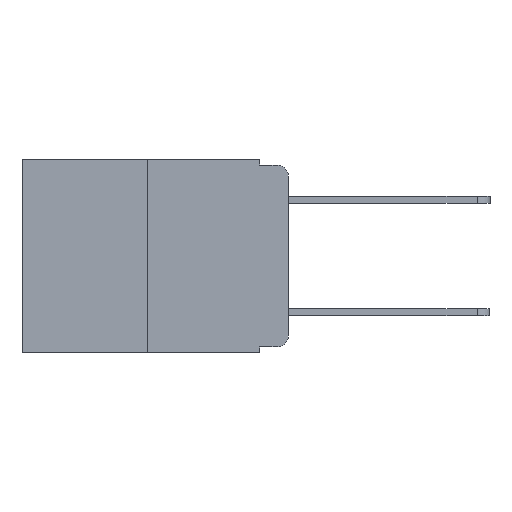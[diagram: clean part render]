
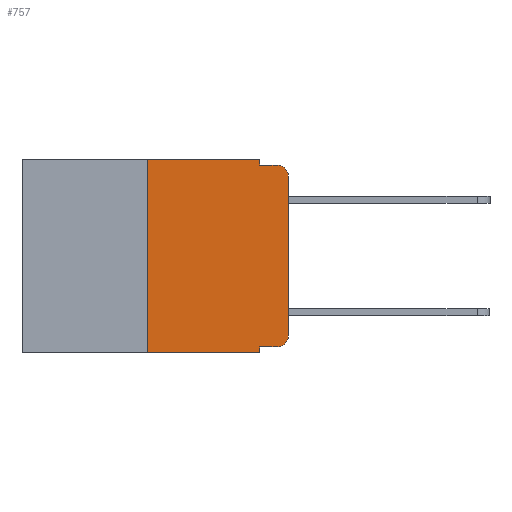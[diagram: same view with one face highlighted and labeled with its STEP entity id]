
A CAD part, left-side view. The second image highlights one B-rep face of the part: STEP entity #757.
In plain terms, the highlighted planar face has unit normal (-1, 0, 0).
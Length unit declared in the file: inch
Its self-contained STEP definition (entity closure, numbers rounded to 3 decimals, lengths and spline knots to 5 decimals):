
#207 = VERTEX_POINT ( 'NONE', #7604 ) ;
#757 = ADVANCED_FACE ( 'NONE', ( #16403 ), #2458, .F. ) ;
#1333 = CARTESIAN_POINT ( 'NONE',  ( 0., 0.02, -0.313 ) ) ;
#1592 = ORIENTED_EDGE ( 'NONE', *, *, #16100, .T. ) ;
#1748 = EDGE_CURVE ( 'NONE', #19135, #207, #5125, .T. ) ;
#2001 = VERTEX_POINT ( 'NONE', #13512 ) ;
#2207 = ORIENTED_EDGE ( 'NONE', *, *, #8407, .F. ) ;
#2458 = PLANE ( 'NONE',  #22875 ) ;
#2484 = AXIS2_PLACEMENT_3D ( 'NONE', #18502, #7836, #20227 ) ;
#2815 = CARTESIAN_POINT ( 'NONE',  ( 0., 0.051, -0.343 ) ) ;
#3214 = DIRECTION ( 'NONE',  ( 0., 0., -1. ) ) ;
#3325 = VECTOR ( 'NONE', #6376, 39.37008 ) ;
#3663 = EDGE_CURVE ( 'NONE', #4426, #10604, #8149, .T. ) ;
#3770 = ORIENTED_EDGE ( 'NONE', *, *, #12910, .T. ) ;
#4057 = LINE ( 'NONE', #16016, #12547 ) ;
#4163 = CIRCLE ( 'NONE', #2484, 0.02 ) ;
#4196 = CARTESIAN_POINT ( 'NONE',  ( 0., 0.25, -0.343 ) ) ;
#4425 = EDGE_CURVE ( 'NONE', #16785, #2001, #16792, .T. ) ;
#4426 = VERTEX_POINT ( 'NONE', #22706 ) ;
#4453 = CARTESIAN_POINT ( 'NONE',  ( 0., 0., -0.03 ) ) ;
#4500 = LINE ( 'NONE', #19977, #8775 ) ;
#4833 = VERTEX_POINT ( 'NONE', #6075 ) ;
#5109 = LINE ( 'NONE', #6701, #14104 ) ;
#5125 = LINE ( 'NONE', #15799, #9956 ) ;
#5719 = DIRECTION ( 'NONE',  ( 0., 0., -1. ) ) ;
#5805 = VECTOR ( 'NONE', #20766, 39.37008 ) ;
#6075 = CARTESIAN_POINT ( 'NONE',  ( 0., 0.02, -0.01 ) ) ;
#6245 = ORIENTED_EDGE ( 'NONE', *, *, #14078, .T. ) ;
#6376 = DIRECTION ( 'NONE',  ( 0., 0., -1. ) ) ;
#6575 = CARTESIAN_POINT ( 'NONE',  ( 0., 0., 0. ) ) ;
#6591 = EDGE_CURVE ( 'NONE', #14006, #4833, #12636, .T. ) ;
#6701 = CARTESIAN_POINT ( 'NONE',  ( 0., 0.473, -0.343 ) ) ;
#6834 = VERTEX_POINT ( 'NONE', #4453 ) ;
#7321 = CARTESIAN_POINT ( 'NONE',  ( 0., 0.051, -0.01 ) ) ;
#7604 = CARTESIAN_POINT ( 'NONE',  ( 0., 0.25, 0. ) ) ;
#7836 = DIRECTION ( 'NONE',  ( -1., 0., 0. ) ) ;
#8149 = LINE ( 'NONE', #17876, #3325 ) ;
#8407 = EDGE_CURVE ( 'NONE', #22431, #14006, #4057, .T. ) ;
#8775 = VECTOR ( 'NONE', #11318, 39.37008 ) ;
#9539 = ORIENTED_EDGE ( 'NONE', *, *, #22775, .F. ) ;
#9803 = CARTESIAN_POINT ( 'NONE',  ( 0., 0.473, 0. ) ) ;
#9956 = VECTOR ( 'NONE', #10819, 39.37008 ) ;
#10178 = EDGE_CURVE ( 'NONE', #19135, #10604, #5109, .T. ) ;
#10604 = VERTEX_POINT ( 'NONE', #2815 ) ;
#10627 = LINE ( 'NONE', #6575, #5805 ) ;
#10819 = DIRECTION ( 'NONE',  ( 0., 0., 1. ) ) ;
#11318 = DIRECTION ( 'NONE',  ( 0., -1., 0. ) ) ;
#11616 = DIRECTION ( 'NONE',  ( 0., -1., 0. ) ) ;
#12024 = ORIENTED_EDGE ( 'NONE', *, *, #3663, .F. ) ;
#12097 = VECTOR ( 'NONE', #12846, 39.37008 ) ;
#12169 = DIRECTION ( 'NONE',  ( 0., -1., 0. ) ) ;
#12547 = VECTOR ( 'NONE', #17937, 39.37008 ) ;
#12636 = LINE ( 'NONE', #7321, #12097 ) ;
#12750 = CARTESIAN_POINT ( 'NONE',  ( 0., 0.051, 0. ) ) ;
#12846 = DIRECTION ( 'NONE',  ( 0., -1., 0. ) ) ;
#12910 = EDGE_CURVE ( 'NONE', #4426, #16785, #4500, .T. ) ;
#12916 = ORIENTED_EDGE ( 'NONE', *, *, #1748, .F. ) ;
#13512 = CARTESIAN_POINT ( 'NONE',  ( 0., 0., -0.313 ) ) ;
#13540 = ORIENTED_EDGE ( 'NONE', *, *, #6591, .F. ) ;
#14005 = DIRECTION ( 'NONE',  ( -1., 0., 0. ) ) ;
#14006 = VERTEX_POINT ( 'NONE', #19926 ) ;
#14078 = EDGE_CURVE ( 'NONE', #6834, #4833, #4163, .T. ) ;
#14104 = VECTOR ( 'NONE', #12169, 39.37008 ) ;
#14227 = ORIENTED_EDGE ( 'NONE', *, *, #4425, .T. ) ;
#15799 = CARTESIAN_POINT ( 'NONE',  ( 0., 0.25, 0. ) ) ;
#16016 = CARTESIAN_POINT ( 'NONE',  ( 0., 0.051, 0. ) ) ;
#16100 = EDGE_CURVE ( 'NONE', #2001, #6834, #10627, .T. ) ;
#16403 = FACE_OUTER_BOUND ( 'NONE', #19066, .T. ) ;
#16785 = VERTEX_POINT ( 'NONE', #21453 ) ;
#16792 = CIRCLE ( 'NONE', #18140, 0.02 ) ;
#17295 = CARTESIAN_POINT ( 'NONE',  ( 0., 0.473, 0. ) ) ;
#17876 = CARTESIAN_POINT ( 'NONE',  ( 0., 0.051, 0. ) ) ;
#17937 = DIRECTION ( 'NONE',  ( 0., 0., -1. ) ) ;
#18140 = AXIS2_PLACEMENT_3D ( 'NONE', #1333, #14005, #3214 ) ;
#18502 = CARTESIAN_POINT ( 'NONE',  ( 0., 0.02, -0.03 ) ) ;
#19066 = EDGE_LOOP ( 'NONE', ( #1592, #6245, #13540, #2207, #9539, #12916, #20565, #12024, #3770, #14227 ) ) ;
#19135 = VERTEX_POINT ( 'NONE', #4196 ) ;
#19926 = CARTESIAN_POINT ( 'NONE',  ( 0., 0.051, -0.01 ) ) ;
#19977 = CARTESIAN_POINT ( 'NONE',  ( 0., 0.051, -0.333 ) ) ;
#20227 = DIRECTION ( 'NONE',  ( 0., 0., -1. ) ) ;
#20565 = ORIENTED_EDGE ( 'NONE', *, *, #10178, .T. ) ;
#20766 = DIRECTION ( 'NONE',  ( 0., 0., 1. ) ) ;
#21453 = CARTESIAN_POINT ( 'NONE',  ( 0., 0.02, -0.333 ) ) ;
#21463 = DIRECTION ( 'NONE',  ( 1., 0., 0. ) ) ;
#22293 = VECTOR ( 'NONE', #11616, 39.37008 ) ;
#22431 = VERTEX_POINT ( 'NONE', #12750 ) ;
#22706 = CARTESIAN_POINT ( 'NONE',  ( 0., 0.051, -0.333 ) ) ;
#22775 = EDGE_CURVE ( 'NONE', #207, #22431, #22842, .T. ) ;
#22842 = LINE ( 'NONE', #9803, #22293 ) ;
#22875 = AXIS2_PLACEMENT_3D ( 'NONE', #17295, #21463, #5719 ) ;
